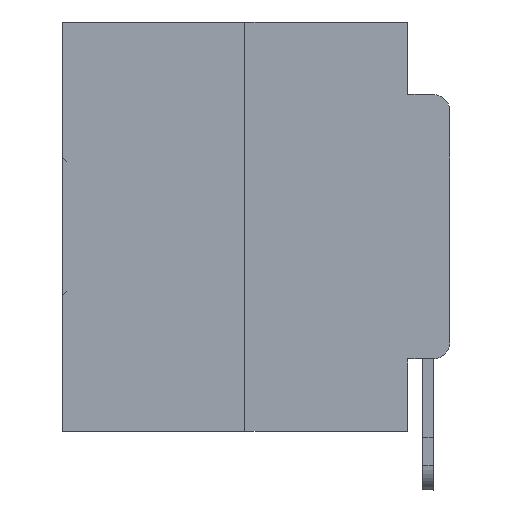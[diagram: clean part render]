
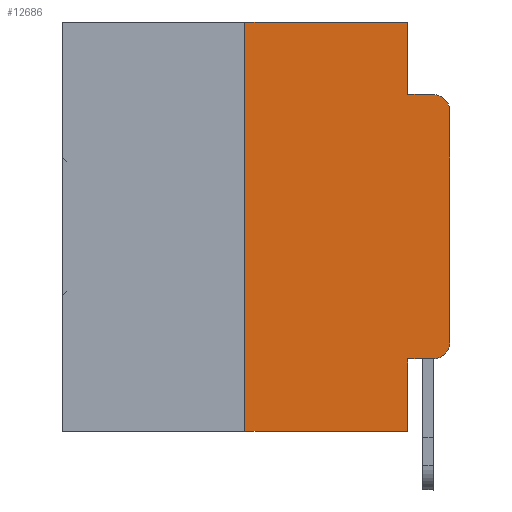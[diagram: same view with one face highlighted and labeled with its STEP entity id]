
A CAD part, left-side view. The second image highlights one B-rep face of the part: STEP entity #12686.
In plain terms, the highlighted planar face has unit normal (-1, 0, 0).
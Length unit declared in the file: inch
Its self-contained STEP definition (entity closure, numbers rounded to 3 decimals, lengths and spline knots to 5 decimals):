
#88 = EDGE_LOOP ( 'NONE', ( #32873, #19181, #25590, #2512, #16409, #28944, #16662, #26747, #31607, #30716 ) ) ;
#337 = DIRECTION ( 'NONE',  ( 0., 0., 1. ) ) ;
#341 = VECTOR ( 'NONE', #4592, 39.37008 ) ;
#482 = CARTESIAN_POINT ( 'NONE',  ( 0., 0.051, 0. ) ) ;
#1432 = DIRECTION ( 'NONE',  ( -1., 0., 0. ) ) ;
#1544 = FACE_OUTER_BOUND ( 'NONE', #88, .T. ) ;
#1781 = EDGE_CURVE ( 'NONE', #4113, #22479, #31966, .T. ) ;
#2256 = CARTESIAN_POINT ( 'NONE',  ( 0., 0.473, -0.5 ) ) ;
#2354 = DIRECTION ( 'NONE',  ( 0., -1., 0. ) ) ;
#2401 = EDGE_CURVE ( 'NONE', #28092, #14303, #9461, .T. ) ;
#2512 = ORIENTED_EDGE ( 'NONE', *, *, #9436, .F. ) ;
#2819 = VECTOR ( 'NONE', #19725, 39.37008 ) ;
#4113 = VERTEX_POINT ( 'NONE', #14678 ) ;
#4299 = LINE ( 'NONE', #12302, #28699 ) ;
#4433 = CARTESIAN_POINT ( 'NONE',  ( 0., 0., -0.1085 ) ) ;
#4473 = CIRCLE ( 'NONE', #5464, 0.02 ) ;
#4592 = DIRECTION ( 'NONE',  ( 0., -1., 0. ) ) ;
#5464 = AXIS2_PLACEMENT_3D ( 'NONE', #14123, #1432, #24338 ) ;
#6303 = CARTESIAN_POINT ( 'NONE',  ( 0., 0.051, 0. ) ) ;
#7130 = EDGE_CURVE ( 'NONE', #15659, #12088, #4299, .T. ) ;
#8032 = LINE ( 'NONE', #6303, #10035 ) ;
#9436 = EDGE_CURVE ( 'NONE', #19964, #15659, #8032, .T. ) ;
#9461 = CIRCLE ( 'NONE', #11063, 0.02 ) ;
#10035 = VECTOR ( 'NONE', #11322, 39.37008 ) ;
#11063 = AXIS2_PLACEMENT_3D ( 'NONE', #25403, #22742, #30252 ) ;
#11322 = DIRECTION ( 'NONE',  ( 0., 0., -1. ) ) ;
#11724 = CARTESIAN_POINT ( 'NONE',  ( 0., 0.473, 0. ) ) ;
#11958 = VECTOR ( 'NONE', #2354, 39.37008 ) ;
#12088 = VERTEX_POINT ( 'NONE', #21636 ) ;
#12302 = CARTESIAN_POINT ( 'NONE',  ( 0., 0.051, -0.0885 ) ) ;
#12686 = ADVANCED_FACE ( 'NONE', ( #1544 ), #22444, .F. ) ;
#13024 = CARTESIAN_POINT ( 'NONE',  ( 0., 0., 0. ) ) ;
#13406 = VERTEX_POINT ( 'NONE', #4433 ) ;
#13590 = VECTOR ( 'NONE', #337, 39.37008 ) ;
#13655 = CARTESIAN_POINT ( 'NONE',  ( 0., 0.051, 0. ) ) ;
#14123 = CARTESIAN_POINT ( 'NONE',  ( 0., 0.02, -0.1085 ) ) ;
#14303 = VERTEX_POINT ( 'NONE', #28920 ) ;
#14618 = LINE ( 'NONE', #2256, #341 ) ;
#14678 = CARTESIAN_POINT ( 'NONE',  ( 0., 0.25, -0.5 ) ) ;
#15056 = LINE ( 'NONE', #17247, #11958 ) ;
#15621 = CARTESIAN_POINT ( 'NONE',  ( 0., 0.25, 0. ) ) ;
#15659 = VERTEX_POINT ( 'NONE', #22579 ) ;
#16409 = ORIENTED_EDGE ( 'NONE', *, *, #24489, .F. ) ;
#16662 = ORIENTED_EDGE ( 'NONE', *, *, #21819, .T. ) ;
#16870 = LINE ( 'NONE', #17208, #2819 ) ;
#16901 = VECTOR ( 'NONE', #24628, 39.37008 ) ;
#17038 = AXIS2_PLACEMENT_3D ( 'NONE', #11724, #29793, #27104 ) ;
#17112 = CARTESIAN_POINT ( 'NONE',  ( 0., 0.25, 0. ) ) ;
#17208 = CARTESIAN_POINT ( 'NONE',  ( 0., 0.051, -0.4115 ) ) ;
#17247 = CARTESIAN_POINT ( 'NONE',  ( 0., 0.473, 0. ) ) ;
#17876 = EDGE_CURVE ( 'NONE', #13406, #12088, #4473, .T. ) ;
#18362 = EDGE_CURVE ( 'NONE', #23662, #28092, #16870, .T. ) ;
#19181 = ORIENTED_EDGE ( 'NONE', *, *, #17876, .T. ) ;
#19725 = DIRECTION ( 'NONE',  ( 0., -1., 0. ) ) ;
#19870 = EDGE_CURVE ( 'NONE', #23662, #24305, #28872, .T. ) ;
#19964 = VERTEX_POINT ( 'NONE', #13655 ) ;
#21636 = CARTESIAN_POINT ( 'NONE',  ( 0., 0.02, -0.0885 ) ) ;
#21819 = EDGE_CURVE ( 'NONE', #4113, #24305, #14618, .T. ) ;
#21921 = CARTESIAN_POINT ( 'NONE',  ( 0., 0.02, -0.4115 ) ) ;
#22123 = VECTOR ( 'NONE', #24036, 39.37008 ) ;
#22444 = PLANE ( 'NONE',  #17038 ) ;
#22479 = VERTEX_POINT ( 'NONE', #15621 ) ;
#22579 = CARTESIAN_POINT ( 'NONE',  ( 0., 0.051, -0.0885 ) ) ;
#22742 = DIRECTION ( 'NONE',  ( -1., 0., 0. ) ) ;
#23416 = EDGE_CURVE ( 'NONE', #14303, #13406, #25740, .T. ) ;
#23662 = VERTEX_POINT ( 'NONE', #32564 ) ;
#24036 = DIRECTION ( 'NONE',  ( 0., 0., -1. ) ) ;
#24305 = VERTEX_POINT ( 'NONE', #24596 ) ;
#24338 = DIRECTION ( 'NONE',  ( 0., 0., -1. ) ) ;
#24489 = EDGE_CURVE ( 'NONE', #22479, #19964, #15056, .T. ) ;
#24530 = DIRECTION ( 'NONE',  ( 0., -1., 0. ) ) ;
#24596 = CARTESIAN_POINT ( 'NONE',  ( 0., 0.051, -0.5 ) ) ;
#24628 = DIRECTION ( 'NONE',  ( 0., 0., 1. ) ) ;
#25403 = CARTESIAN_POINT ( 'NONE',  ( 0., 0.02, -0.3915 ) ) ;
#25590 = ORIENTED_EDGE ( 'NONE', *, *, #7130, .F. ) ;
#25740 = LINE ( 'NONE', #13024, #13590 ) ;
#26747 = ORIENTED_EDGE ( 'NONE', *, *, #19870, .F. ) ;
#27104 = DIRECTION ( 'NONE',  ( 0., 0., -1. ) ) ;
#28092 = VERTEX_POINT ( 'NONE', #21921 ) ;
#28699 = VECTOR ( 'NONE', #24530, 39.37008 ) ;
#28872 = LINE ( 'NONE', #482, #22123 ) ;
#28920 = CARTESIAN_POINT ( 'NONE',  ( 0., 0., -0.3915 ) ) ;
#28944 = ORIENTED_EDGE ( 'NONE', *, *, #1781, .F. ) ;
#29793 = DIRECTION ( 'NONE',  ( 1., 0., 0. ) ) ;
#30252 = DIRECTION ( 'NONE',  ( 0., 0., -1. ) ) ;
#30716 = ORIENTED_EDGE ( 'NONE', *, *, #2401, .T. ) ;
#31607 = ORIENTED_EDGE ( 'NONE', *, *, #18362, .T. ) ;
#31966 = LINE ( 'NONE', #17112, #16901 ) ;
#32564 = CARTESIAN_POINT ( 'NONE',  ( 0., 0.051, -0.4115 ) ) ;
#32873 = ORIENTED_EDGE ( 'NONE', *, *, #23416, .T. ) ;
